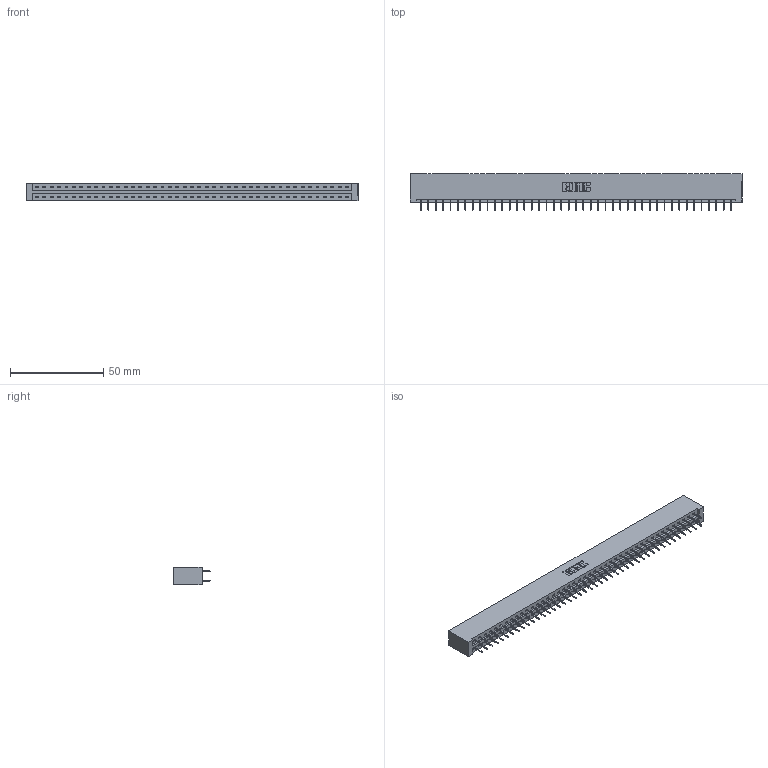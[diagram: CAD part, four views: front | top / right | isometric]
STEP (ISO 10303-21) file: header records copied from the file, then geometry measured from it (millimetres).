
FILE_DESCRIPTION (( 'STEP AP203' ), '1' );
FILE_NAME ('387-086-524-201.STEP', '2019-10-23T03:11:09', ( '' ), ( '' ), 'SwSTEP 2.0', 'SolidWorks 2016', '' );
FILE_SCHEMA (( 'CONFIG_CONTROL_DESIGN' ));
Length unit declared in the file: inch
Products named in the file (3): 345-292-001_345-293-124; 387-086-524-201; 337 Part_No Mounting Lugs
Assembly tree (87 placements, depth 2):
  387-086-524-201
    337 Part_No Mounting Lugs
    345-292-001_345-293-124  x86
Bounding box: 178.26 x 19.69 x 9.4 mm (x, y, z)
Volume: 19430.1 mm3; surface area: 21628.5 mm2
Topology: 87 solids, 87 shells, 5094 faces, 14477 edges, 9306 vertices
Faces by surface type: plane 3850, cylinder 1244
Entity records: 33007 total; most frequent: CARTESIAN_POINT 5558, ORIENTED_EDGE 5494, DIRECTION 4719, EDGE_CURVE 2747, VECTOR 2631, LINE 2631, VERTEX_POINT 1826, AXIS2_PLACEMENT_3D 1044
